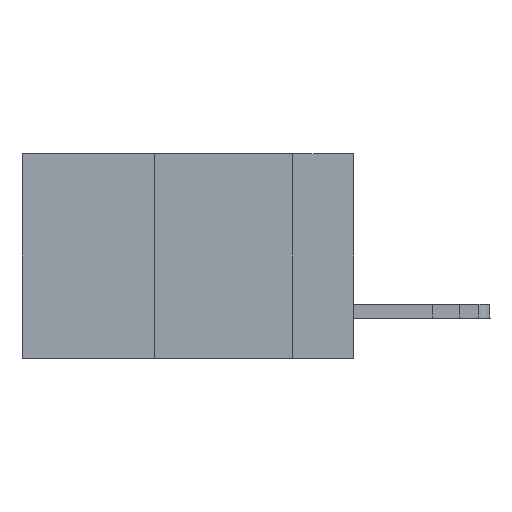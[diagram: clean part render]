
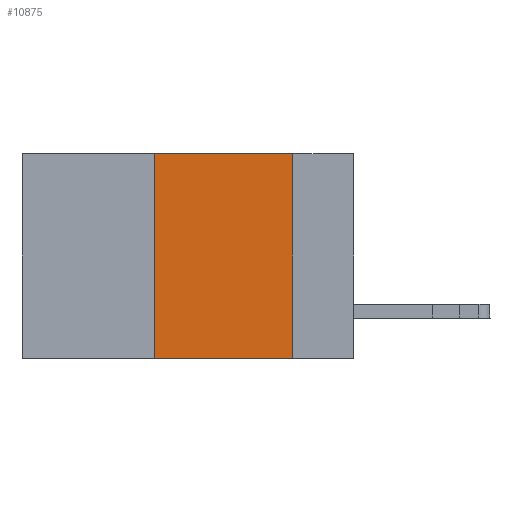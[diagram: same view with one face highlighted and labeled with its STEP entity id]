
A CAD part, left-side view. The second image highlights one B-rep face of the part: STEP entity #10875.
In plain terms, the highlighted planar face has unit normal (-1, 0, 0).
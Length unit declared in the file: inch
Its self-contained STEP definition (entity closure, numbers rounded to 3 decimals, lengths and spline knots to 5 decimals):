
#249 = ORIENTED_EDGE ( 'NONE', *, *, #7699, .T. ) ;
#353 = VECTOR ( 'NONE', #18848, 39.37008 ) ;
#857 = VECTOR ( 'NONE', #9738, 39.37008 ) ;
#1629 = VERTEX_POINT ( 'NONE', #11927 ) ;
#1721 = CARTESIAN_POINT ( 'NONE',  ( 0., 0.36, 0. ) ) ;
#2442 = CARTESIAN_POINT ( 'NONE',  ( 0., 0.36, 0. ) ) ;
#2510 = EDGE_CURVE ( 'NONE', #2696, #6730, #13688, .T. ) ;
#2696 = VERTEX_POINT ( 'NONE', #1721 ) ;
#3423 = EDGE_CURVE ( 'NONE', #6730, #1629, #8310, .T. ) ;
#3725 = CARTESIAN_POINT ( 'NONE',  ( 0., 0.11, 0. ) ) ;
#3961 = DIRECTION ( 'NONE',  ( 1., 0., 0. ) ) ;
#4333 = FACE_OUTER_BOUND ( 'NONE', #7981, .T. ) ;
#4727 = VERTEX_POINT ( 'NONE', #9491 ) ;
#4852 = VECTOR ( 'NONE', #15440, 39.37008 ) ;
#5209 = DIRECTION ( 'NONE',  ( 0., 0., -1. ) ) ;
#6164 = LINE ( 'NONE', #2442, #353 ) ;
#6730 = VERTEX_POINT ( 'NONE', #3725 ) ;
#6897 = CARTESIAN_POINT ( 'NONE',  ( 0., 0.11, 0. ) ) ;
#7154 = DIRECTION ( 'NONE',  ( 0., -1., 0. ) ) ;
#7699 = EDGE_CURVE ( 'NONE', #4727, #1629, #15037, .T. ) ;
#7760 = CARTESIAN_POINT ( 'NONE',  ( 0., 0.6, -0.37 ) ) ;
#7981 = EDGE_LOOP ( 'NONE', ( #18816, #10876, #16469, #249 ) ) ;
#8310 = LINE ( 'NONE', #6897, #857 ) ;
#9491 = CARTESIAN_POINT ( 'NONE',  ( 0., 0.36, -0.37 ) ) ;
#9596 = CARTESIAN_POINT ( 'NONE',  ( 0., 0.6, 0. ) ) ;
#9738 = DIRECTION ( 'NONE',  ( 0., 0., -1. ) ) ;
#9869 = CARTESIAN_POINT ( 'NONE',  ( 0., 0.6, 0. ) ) ;
#10875 = ADVANCED_FACE ( 'NONE', ( #4333 ), #14225, .F. ) ;
#10876 = ORIENTED_EDGE ( 'NONE', *, *, #2510, .F. ) ;
#10911 = VECTOR ( 'NONE', #7154, 39.37008 ) ;
#11927 = CARTESIAN_POINT ( 'NONE',  ( 0., 0.11, -0.37 ) ) ;
#12027 = EDGE_CURVE ( 'NONE', #4727, #2696, #6164, .T. ) ;
#13688 = LINE ( 'NONE', #9596, #4852 ) ;
#14225 = PLANE ( 'NONE',  #17145 ) ;
#15037 = LINE ( 'NONE', #7760, #10911 ) ;
#15440 = DIRECTION ( 'NONE',  ( 0., -1., 0. ) ) ;
#16469 = ORIENTED_EDGE ( 'NONE', *, *, #12027, .F. ) ;
#17145 = AXIS2_PLACEMENT_3D ( 'NONE', #9869, #3961, #5209 ) ;
#18816 = ORIENTED_EDGE ( 'NONE', *, *, #3423, .F. ) ;
#18848 = DIRECTION ( 'NONE',  ( 0., 0., 1. ) ) ;
